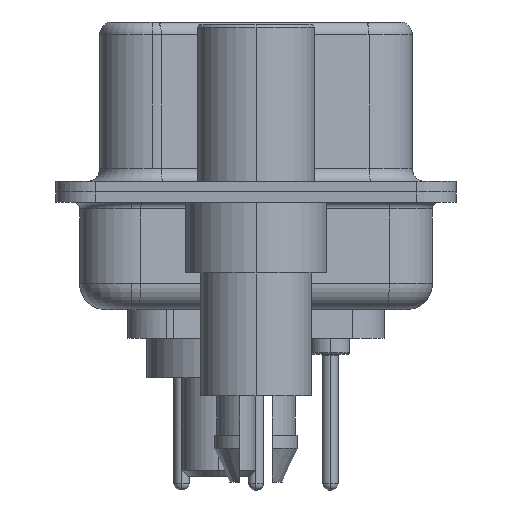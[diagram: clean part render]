
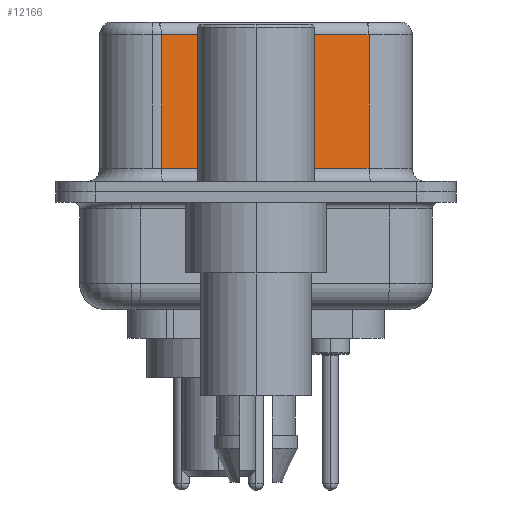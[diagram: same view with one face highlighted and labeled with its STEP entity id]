
A CAD part, left-side view. The second image highlights one B-rep face of the part: STEP entity #12166.
In plain terms, the highlighted planar face has unit normal (-0.985, -0.174, 0).
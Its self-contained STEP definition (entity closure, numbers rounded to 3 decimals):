
#1178 = DIRECTION ( 'NONE',  ( -0.174, 0.985, 0. ) ) ;
#1329 = DIRECTION ( 'NONE',  ( -0.174, 0.985, 0. ) ) ;
#2071 = CARTESIAN_POINT ( 'NONE',  ( 3.73, 3.628, 6.02 ) ) ;
#2308 = DIRECTION ( 'NONE',  ( 0., 0., -1. ) ) ;
#3350 = VERTEX_POINT ( 'NONE', #12685 ) ;
#3457 = PLANE ( 'NONE',  #19154 ) ;
#4735 = LINE ( 'NONE', #25787, #15071 ) ;
#4757 = VECTOR ( 'NONE', #2308, 1000. ) ;
#4980 = ORIENTED_EDGE ( 'NONE', *, *, #25010, .T. ) ;
#5064 = ORIENTED_EDGE ( 'NONE', *, *, #7716, .T. ) ;
#5338 = VECTOR ( 'NONE', #7498, 1000. ) ;
#5457 = CARTESIAN_POINT ( 'NONE',  ( 3.73, 3.628, 6.52 ) ) ;
#5952 = LINE ( 'NONE', #5457, #5338 ) ;
#7089 = VERTEX_POINT ( 'NONE', #21855 ) ;
#7498 = DIRECTION ( 'NONE',  ( 0., 0., -1. ) ) ;
#7716 = EDGE_CURVE ( 'NONE', #22899, #3350, #10351, .T. ) ;
#9665 = CARTESIAN_POINT ( 'NONE',  ( 5.132, -4.322, 6.52 ) ) ;
#10334 = CARTESIAN_POINT ( 'NONE',  ( 3.73, 3.628, 0.9 ) ) ;
#10351 = LINE ( 'NONE', #22015, #15878 ) ;
#10643 = CARTESIAN_POINT ( 'NONE',  ( 5.132, -4.322, 6.52 ) ) ;
#12166 = ADVANCED_FACE ( 'NONE', ( #23963 ), #3457, .F. ) ;
#12685 = CARTESIAN_POINT ( 'NONE',  ( 5.132, -4.322, 0.9 ) ) ;
#13843 = DIRECTION ( 'NONE',  ( 0.985, 0.174, 0. ) ) ;
#15071 = VECTOR ( 'NONE', #1178, 1000. ) ;
#15281 = EDGE_CURVE ( 'NONE', #7089, #21216, #4735, .T. ) ;
#15878 = VECTOR ( 'NONE', #17972, 1000. ) ;
#17972 = DIRECTION ( 'NONE',  ( 0.174, -0.985, 0. ) ) ;
#18766 = ORIENTED_EDGE ( 'NONE', *, *, #24089, .F. ) ;
#19154 = AXIS2_PLACEMENT_3D ( 'NONE', #9665, #13843, #1329 ) ;
#20447 = LINE ( 'NONE', #10643, #4757 ) ;
#20684 = EDGE_LOOP ( 'NONE', ( #18766, #21325, #4980, #5064 ) ) ;
#21216 = VERTEX_POINT ( 'NONE', #2071 ) ;
#21325 = ORIENTED_EDGE ( 'NONE', *, *, #15281, .T. ) ;
#21855 = CARTESIAN_POINT ( 'NONE',  ( 5.132, -4.322, 6.02 ) ) ;
#22015 = CARTESIAN_POINT ( 'NONE',  ( 5.132, -4.322, 0.9 ) ) ;
#22899 = VERTEX_POINT ( 'NONE', #10334 ) ;
#23963 = FACE_OUTER_BOUND ( 'NONE', #20684, .T. ) ;
#24089 = EDGE_CURVE ( 'NONE', #7089, #3350, #20447, .T. ) ;
#25010 = EDGE_CURVE ( 'NONE', #21216, #22899, #5952, .T. ) ;
#25787 = CARTESIAN_POINT ( 'NONE',  ( 5.132, -4.322, 6.02 ) ) ;
